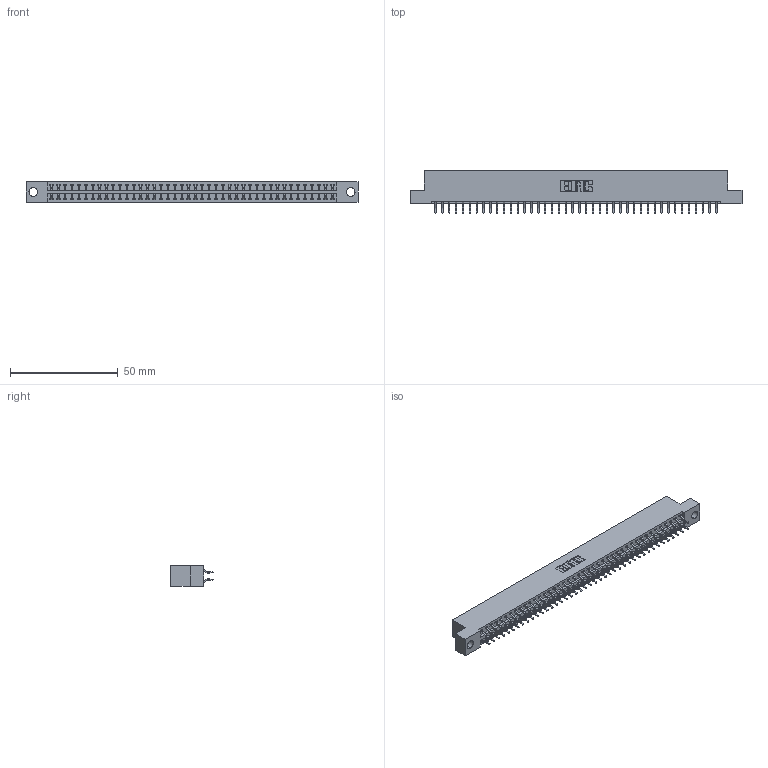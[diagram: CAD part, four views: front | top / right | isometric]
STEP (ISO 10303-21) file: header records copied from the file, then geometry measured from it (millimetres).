
FILE_DESCRIPTION (( 'STEP AP203' ), '1' );
FILE_NAME ('396-084-556-204.STEP', '2018-09-10T01:37:32', ( '' ), ( '' ), 'SwSTEP 2.0', 'SolidWorks 2016', '' );
FILE_SCHEMA (( 'CONFIG_CONTROL_DESIGN' ));
Length unit declared in the file: inch
Products named in the file (3): 346 Part_Flush Mounting Lugs - 0.156 Dia-TH; 345-292-001_556 Tail; 396-084-556-204
Assembly tree (85 placements, depth 2):
  396-084-556-204
    346 Part_Flush Mounting Lugs - 0.156 Dia-TH
    345-292-001_556 Tail  x84
Bounding box: 153.92 x 19.57 x 9.4 mm (x, y, z)
Volume: 14918.3 mm3; surface area: 20241.6 mm2
Topology: 85 solids, 85 shells, 4994 faces, 14861 edges, 9794 vertices
Faces by surface type: plane 3352, cylinder 1642
Entity records: 27633 total; most frequent: CARTESIAN_POINT 4568, ORIENTED_EDGE 4490, DIRECTION 4065, EDGE_CURVE 2245, VECTOR 1937, LINE 1937, VERTEX_POINT 1494, AXIS2_PLACEMENT_3D 1064
